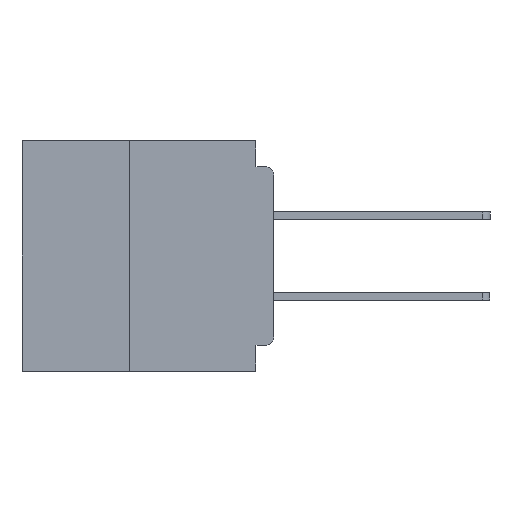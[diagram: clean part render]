
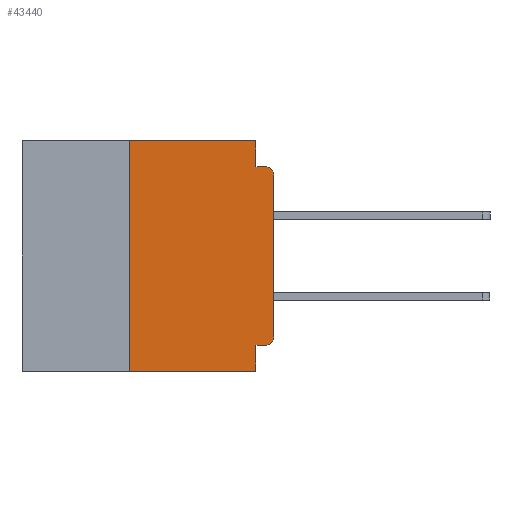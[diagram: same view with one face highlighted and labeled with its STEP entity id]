
A CAD part, left-side view. The second image highlights one B-rep face of the part: STEP entity #43440.
In plain terms, the highlighted planar face has unit normal (-1, 0, 0).
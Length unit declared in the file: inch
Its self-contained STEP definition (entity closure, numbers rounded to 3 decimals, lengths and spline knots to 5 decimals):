
#29 = AXIS2_PLACEMENT_3D ( 'NONE', #28679, #8434, #32050 ) ;
#623 = CARTESIAN_POINT ( 'NONE',  ( 0., 0.031, -0.045 ) ) ;
#896 = VECTOR ( 'NONE', #21493, 39.37008 ) ;
#1098 = DIRECTION ( 'NONE',  ( 0., 0., -1. ) ) ;
#1421 = ORIENTED_EDGE ( 'NONE', *, *, #7282, .T. ) ;
#1944 = VECTOR ( 'NONE', #39604, 39.37008 ) ;
#2488 = EDGE_CURVE ( 'NONE', #15194, #24973, #19056, .T. ) ;
#4336 = VECTOR ( 'NONE', #43624, 39.37008 ) ;
#4584 = CARTESIAN_POINT ( 'NONE',  ( 0., 0.437, 0. ) ) ;
#4776 = ORIENTED_EDGE ( 'NONE', *, *, #17672, .F. ) ;
#4792 = EDGE_CURVE ( 'NONE', #13072, #35982, #39340, .T. ) ;
#4830 = CARTESIAN_POINT ( 'NONE',  ( 0., 0., -0.355 ) ) ;
#4875 = VECTOR ( 'NONE', #32342, 39.37008 ) ;
#5093 = EDGE_CURVE ( 'NONE', #12525, #32698, #26764, .T. ) ;
#5240 = DIRECTION ( 'NONE',  ( 0., 1., 0. ) ) ;
#5722 = CARTESIAN_POINT ( 'NONE',  ( 0., 0.031, 0. ) ) ;
#5935 = LINE ( 'NONE', #28977, #4875 ) ;
#6026 = CARTESIAN_POINT ( 'NONE',  ( 0., 0.031, -0.4 ) ) ;
#7282 = EDGE_CURVE ( 'NONE', #12525, #35566, #11725, .T. ) ;
#8052 = EDGE_CURVE ( 'NONE', #35566, #43128, #5935, .T. ) ;
#8434 = DIRECTION ( 'NONE',  ( -1., 0., 0. ) ) ;
#9011 = VECTOR ( 'NONE', #43328, 39.37008 ) ;
#10670 = EDGE_LOOP ( 'NONE', ( #27454, #34437, #4776, #13835, #34676, #14436, #41553, #18006, #11870, #1421 ) ) ;
#10830 = DIRECTION ( 'NONE',  ( 0., -1., 0. ) ) ;
#10880 = CARTESIAN_POINT ( 'NONE',  ( 0., 0.437, -0.4 ) ) ;
#11725 = CIRCLE ( 'NONE', #18180, 0.015 ) ;
#11870 = ORIENTED_EDGE ( 'NONE', *, *, #5093, .F. ) ;
#11977 = CARTESIAN_POINT ( 'NONE',  ( 0., 0.25, -0.4 ) ) ;
#12525 = VERTEX_POINT ( 'NONE', #26232 ) ;
#13072 = VERTEX_POINT ( 'NONE', #11977 ) ;
#13190 = CARTESIAN_POINT ( 'NONE',  ( 0., 0.015, -0.045 ) ) ;
#13835 = ORIENTED_EDGE ( 'NONE', *, *, #2488, .F. ) ;
#14436 = ORIENTED_EDGE ( 'NONE', *, *, #16899, .F. ) ;
#15194 = VERTEX_POINT ( 'NONE', #5722 ) ;
#16271 = CARTESIAN_POINT ( 'NONE',  ( 0., 0.25, 0. ) ) ;
#16899 = EDGE_CURVE ( 'NONE', #13072, #17553, #17102, .T. ) ;
#17102 = LINE ( 'NONE', #26247, #25093 ) ;
#17208 = CARTESIAN_POINT ( 'NONE',  ( 0., 0.031, 0. ) ) ;
#17553 = VERTEX_POINT ( 'NONE', #16271 ) ;
#17638 = FACE_OUTER_BOUND ( 'NONE', #10670, .T. ) ;
#17672 = EDGE_CURVE ( 'NONE', #24973, #35737, #23431, .T. ) ;
#17744 = VECTOR ( 'NONE', #5240, 39.37008 ) ;
#17924 = CIRCLE ( 'NONE', #29, 0.015 ) ;
#18006 = ORIENTED_EDGE ( 'NONE', *, *, #41019, .F. ) ;
#18079 = DIRECTION ( 'NONE',  ( 1., 0., 0. ) ) ;
#18180 = AXIS2_PLACEMENT_3D ( 'NONE', #41506, #21394, #1098 ) ;
#19056 = LINE ( 'NONE', #17208, #9011 ) ;
#21394 = DIRECTION ( 'NONE',  ( -1., 0., 0. ) ) ;
#21493 = DIRECTION ( 'NONE',  ( 0., -1., 0. ) ) ;
#23431 = LINE ( 'NONE', #30275, #4336 ) ;
#24085 = CARTESIAN_POINT ( 'NONE',  ( 0., 0.031, -0.355 ) ) ;
#24973 = VERTEX_POINT ( 'NONE', #623 ) ;
#25093 = VECTOR ( 'NONE', #29617, 39.37008 ) ;
#26232 = CARTESIAN_POINT ( 'NONE',  ( 0., 0.015, -0.355 ) ) ;
#26247 = CARTESIAN_POINT ( 'NONE',  ( 0., 0.25, -0.4 ) ) ;
#26764 = LINE ( 'NONE', #4830, #17744 ) ;
#27454 = ORIENTED_EDGE ( 'NONE', *, *, #8052, .T. ) ;
#28250 = CARTESIAN_POINT ( 'NONE',  ( 0., 0.031, -0.4 ) ) ;
#28679 = CARTESIAN_POINT ( 'NONE',  ( 0., 0.015, -0.06 ) ) ;
#28977 = CARTESIAN_POINT ( 'NONE',  ( 0., 0., 0. ) ) ;
#29617 = DIRECTION ( 'NONE',  ( 0., 0., 1. ) ) ;
#29968 = LINE ( 'NONE', #6026, #1944 ) ;
#30275 = CARTESIAN_POINT ( 'NONE',  ( 0., 0., -0.045 ) ) ;
#31333 = AXIS2_PLACEMENT_3D ( 'NONE', #38224, #18079, #41624 ) ;
#31518 = VECTOR ( 'NONE', #10830, 39.37008 ) ;
#31694 = EDGE_CURVE ( 'NONE', #17553, #15194, #36791, .T. ) ;
#32050 = DIRECTION ( 'NONE',  ( 0., 0., -1. ) ) ;
#32342 = DIRECTION ( 'NONE',  ( 0., 0., 1. ) ) ;
#32698 = VERTEX_POINT ( 'NONE', #24085 ) ;
#33289 = CARTESIAN_POINT ( 'NONE',  ( 0., 0., -0.06 ) ) ;
#34437 = ORIENTED_EDGE ( 'NONE', *, *, #39666, .T. ) ;
#34676 = ORIENTED_EDGE ( 'NONE', *, *, #31694, .F. ) ;
#34862 = PLANE ( 'NONE',  #31333 ) ;
#35566 = VERTEX_POINT ( 'NONE', #39385 ) ;
#35737 = VERTEX_POINT ( 'NONE', #13190 ) ;
#35982 = VERTEX_POINT ( 'NONE', #28250 ) ;
#36791 = LINE ( 'NONE', #4584, #896 ) ;
#38224 = CARTESIAN_POINT ( 'NONE',  ( 0., 0.437, 0. ) ) ;
#39340 = LINE ( 'NONE', #10880, #31518 ) ;
#39385 = CARTESIAN_POINT ( 'NONE',  ( 0., 0., -0.34 ) ) ;
#39604 = DIRECTION ( 'NONE',  ( 0., 0., -1. ) ) ;
#39666 = EDGE_CURVE ( 'NONE', #43128, #35737, #17924, .T. ) ;
#41019 = EDGE_CURVE ( 'NONE', #32698, #35982, #29968, .T. ) ;
#41506 = CARTESIAN_POINT ( 'NONE',  ( 0., 0.015, -0.34 ) ) ;
#41553 = ORIENTED_EDGE ( 'NONE', *, *, #4792, .T. ) ;
#41624 = DIRECTION ( 'NONE',  ( 0., 0., -1. ) ) ;
#43128 = VERTEX_POINT ( 'NONE', #33289 ) ;
#43328 = DIRECTION ( 'NONE',  ( 0., 0., -1. ) ) ;
#43440 = ADVANCED_FACE ( 'NONE', ( #17638 ), #34862, .F. ) ;
#43624 = DIRECTION ( 'NONE',  ( 0., -1., 0. ) ) ;
